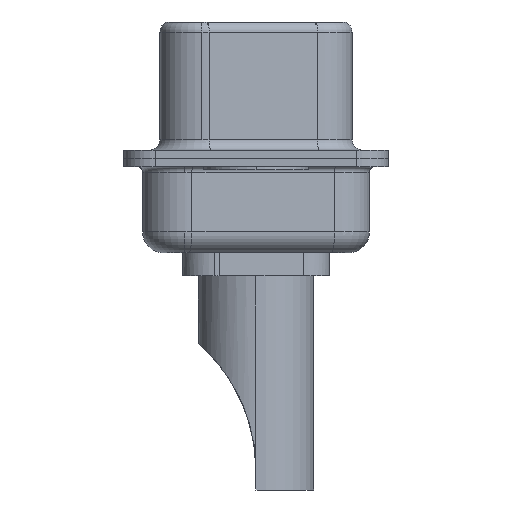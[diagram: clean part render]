
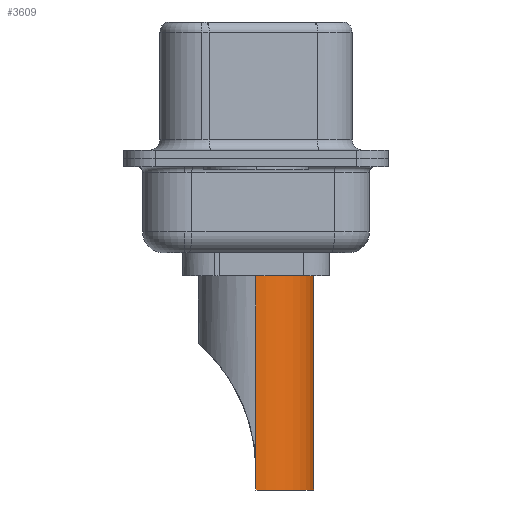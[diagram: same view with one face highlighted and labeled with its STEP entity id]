
A CAD part, left-side view. The second image highlights one B-rep face of the part: STEP entity #3609.
In plain terms, the highlighted cylindrical face has radius 2.75 mm (diameter 5.5 mm), a partial arc.
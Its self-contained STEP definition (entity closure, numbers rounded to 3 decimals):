
#534 = ORIENTED_EDGE ( 'NONE', *, *, #14904, .F. ) ;
#641 = DIRECTION ( 'NONE',  ( 0., 0., -1. ) ) ;
#1324 = DIRECTION ( 'NONE',  ( 1., 0., 0. ) ) ;
#1671 = VERTEX_POINT ( 'NONE', #11998 ) ;
#1814 = VECTOR ( 'NONE', #7894, 1000. ) ;
#3014 = CARTESIAN_POINT ( 'NONE',  ( -2.75, 0., -8.7 ) ) ;
#3434 = EDGE_CURVE ( 'NONE', #12729, #19333, #11667, .T. ) ;
#3519 = AXIS2_PLACEMENT_3D ( 'NONE', #3849, #14573, #13017 ) ;
#3609 = ADVANCED_FACE ( 'NONE', ( #12868 ), #8292, .T. ) ;
#3793 = ORIENTED_EDGE ( 'NONE', *, *, #9673, .T. ) ;
#3849 = CARTESIAN_POINT ( 'NONE',  ( 0., 0., 4.234 ) ) ;
#5295 = CARTESIAN_POINT ( 'NONE',  ( 2.75, 0., 1.5 ) ) ;
#6594 = DIRECTION ( 'NONE',  ( 0., 0., 1. ) ) ;
#6744 = CARTESIAN_POINT ( 'NONE',  ( 0., 0., 1.5 ) ) ;
#7602 = VECTOR ( 'NONE', #6594, 1000. ) ;
#7685 = VERTEX_POINT ( 'NONE', #11007 ) ;
#7894 = DIRECTION ( 'NONE',  ( 0., 0., 1. ) ) ;
#8263 = DIRECTION ( 'NONE',  ( 1., 0., 0. ) ) ;
#8292 = CYLINDRICAL_SURFACE ( 'NONE', #3519, 2.75 ) ;
#8305 = AXIS2_PLACEMENT_3D ( 'NONE', #6744, #17475, #8263 ) ;
#9673 = EDGE_CURVE ( 'NONE', #1671, #17356, #17931, .T. ) ;
#9973 = EDGE_CURVE ( 'NONE', #16118, #19333, #13121, .T. ) ;
#10496 = DIRECTION ( 'NONE',  ( 0., 0., 1. ) ) ;
#10551 = ORIENTED_EDGE ( 'NONE', *, *, #9973, .F. ) ;
#10558 = CARTESIAN_POINT ( 'NONE',  ( -2.75, 0., -8.7 ) ) ;
#10719 = ORIENTED_EDGE ( 'NONE', *, *, #3434, .T. ) ;
#10901 = EDGE_CURVE ( 'NONE', #1671, #16118, #14047, .T. ) ;
#11007 = CARTESIAN_POINT ( 'NONE',  ( 2.75, 0., -8.7 ) ) ;
#11667 = LINE ( 'NONE', #15777, #7602 ) ;
#11671 = CARTESIAN_POINT ( 'NONE',  ( 2.75, 0., -7.764 ) ) ;
#11724 = AXIS2_PLACEMENT_3D ( 'NONE', #19732, #10496, #1324 ) ;
#11998 = CARTESIAN_POINT ( 'NONE',  ( -2.75, 0., -7.764 ) ) ;
#12729 = VERTEX_POINT ( 'NONE', #11671 ) ;
#12868 = FACE_OUTER_BOUND ( 'NONE', #19220, .T. ) ;
#13017 = DIRECTION ( 'NONE',  ( 1., 0., 0. ) ) ;
#13121 = CIRCLE ( 'NONE', #8305, 2.75 ) ;
#13712 = DIRECTION ( 'NONE',  ( 0., 0., -1. ) ) ;
#14047 = LINE ( 'NONE', #17086, #1814 ) ;
#14333 = VECTOR ( 'NONE', #13712, 1000. ) ;
#14573 = DIRECTION ( 'NONE',  ( 0., 0., 1. ) ) ;
#14904 = EDGE_CURVE ( 'NONE', #12729, #7685, #15948, .T. ) ;
#15473 = VECTOR ( 'NONE', #641, 1000. ) ;
#15777 = CARTESIAN_POINT ( 'NONE',  ( 2.75, 0., 4.234 ) ) ;
#15948 = LINE ( 'NONE', #19046, #15473 ) ;
#16118 = VERTEX_POINT ( 'NONE', #17863 ) ;
#16464 = ORIENTED_EDGE ( 'NONE', *, *, #10901, .F. ) ;
#17086 = CARTESIAN_POINT ( 'NONE',  ( -2.75, 0., 4.234 ) ) ;
#17356 = VERTEX_POINT ( 'NONE', #10558 ) ;
#17475 = DIRECTION ( 'NONE',  ( 0., 0., 1. ) ) ;
#17579 = ORIENTED_EDGE ( 'NONE', *, *, #19567, .T. ) ;
#17863 = CARTESIAN_POINT ( 'NONE',  ( -2.75, 0., 1.5 ) ) ;
#17931 = LINE ( 'NONE', #3014, #14333 ) ;
#19046 = CARTESIAN_POINT ( 'NONE',  ( 2.75, 0., -8.7 ) ) ;
#19220 = EDGE_LOOP ( 'NONE', ( #16464, #3793, #17579, #534, #10719, #10551 ) ) ;
#19333 = VERTEX_POINT ( 'NONE', #5295 ) ;
#19351 = CIRCLE ( 'NONE', #11724, 2.75 ) ;
#19567 = EDGE_CURVE ( 'NONE', #17356, #7685, #19351, .T. ) ;
#19732 = CARTESIAN_POINT ( 'NONE',  ( 0., 0., -8.7 ) ) ;
